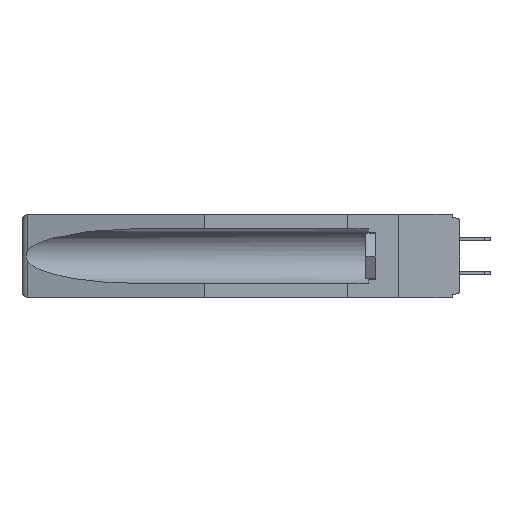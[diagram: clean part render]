
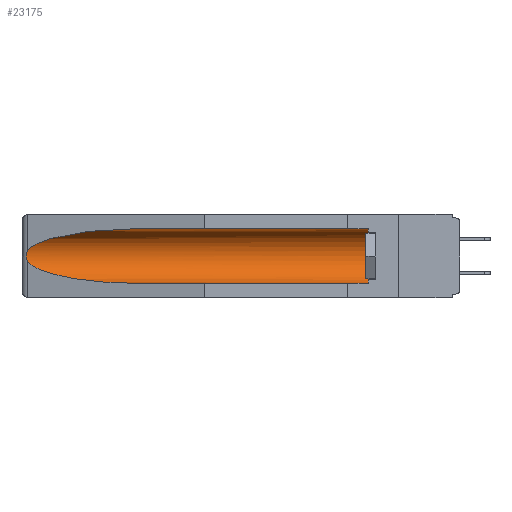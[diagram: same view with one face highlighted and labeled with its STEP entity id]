
A CAD part, left-side view. The second image highlights one B-rep face of the part: STEP entity #23175.
In plain terms, the highlighted cylindrical face has radius 2.857 mm (diameter 5.715 mm), a partial arc.
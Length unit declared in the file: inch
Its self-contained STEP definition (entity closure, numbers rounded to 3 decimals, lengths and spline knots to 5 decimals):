
#35 =( BOUNDED_CURVE ( )  B_SPLINE_CURVE ( 3, ( #17990, #20136, #7535, #20495 ),
 .UNSPECIFIED., .F., .F. ) 
 B_SPLINE_CURVE_WITH_KNOTS ( ( 4, 4 ),
 ( 4.71239, 6.08839 ),
 .UNSPECIFIED. ) 
 CURVE ( )  GEOMETRIC_REPRESENTATION_ITEM ( )  RATIONAL_B_SPLINE_CURVE ( ( 1., 0.848, 0.848, 1. ) ) 
 REPRESENTATION_ITEM ( '' )  );
#2315 = DIRECTION ( 'NONE',  ( 0., 1., 0. ) ) ;
#2699 = CARTESIAN_POINT ( 'NONE',  ( 0.155, -0.30754, -0.1715 ) ) ;
#2771 = ORIENTED_EDGE ( 'NONE', *, *, #7260, .F. ) ;
#3774 = CARTESIAN_POINT ( 'NONE',  ( 0.26654, 1.53092, -0.15636 ) ) ;
#4190 = CARTESIAN_POINT ( 'NONE',  ( 0.26537, 1.52718, -0.14972 ) ) ;
#4200 = CARTESIAN_POINT ( 'NONE',  ( 0.21114, 1.30732, -0.284 ) ) ;
#4686 = ORIENTED_EDGE ( 'NONE', *, *, #25922, .T. ) ;
#4822 = CARTESIAN_POINT ( 'NONE',  ( 0.155, -0.30754, -0.284 ) ) ;
#5340 = EDGE_CURVE ( 'NONE', #10968, #17096, #16891, .T. ) ;
#6312 = LINE ( 'NONE', #21049, #22371 ) ;
#6696 = DIRECTION ( 'NONE',  ( 0., 0., 1. ) ) ;
#7186 = CARTESIAN_POINT ( 'NONE',  ( 0.155, 1.07973, -0.284 ) ) ;
#7260 = EDGE_CURVE ( 'NONE', #10968, #26595, #7734, .T. ) ;
#7535 = CARTESIAN_POINT ( 'NONE',  ( 0.25451, 1.48313, -0.09465 ) ) ;
#7734 = LINE ( 'NONE', #4822, #17746 ) ;
#7871 = CARTESIAN_POINT ( 'NONE',  ( 0.26537, 1.52718, -0.19328 ) ) ;
#7887 = EDGE_CURVE ( 'NONE', #22178, #26595, #15762, .T. ) ;
#8467 = VERTEX_POINT ( 'NONE', #10726 ) ;
#8625 = DIRECTION ( 'NONE',  ( 0., -1., 0. ) ) ;
#9494 = CARTESIAN_POINT ( 'NONE',  ( 0.26597, 1.52961, -0.15275 ) ) ;
#9852 = EDGE_CURVE ( 'NONE', #17096, #8467, #6312, .T. ) ;
#9952 = B_SPLINE_CURVE_WITH_KNOTS ( 'NONE', 3,
 ( #18239, #9494, #3774, #18697, #12110, #27044, #20656, #14518, #16391, #7871 ),
 .UNSPECIFIED., .F., .F.,
 ( 4, 2, 2, 2, 4 ),
 ( 0., 0.00029, 0.00058, 0.00087, 0.00117 ),
 .UNSPECIFIED. ) ;
#10150 = CYLINDRICAL_SURFACE ( 'NONE', #16971, 0.1125 ) ;
#10726 = CARTESIAN_POINT ( 'NONE',  ( 0.155, 1.07973, -0.059 ) ) ;
#10968 = VERTEX_POINT ( 'NONE', #15198 ) ;
#12110 = CARTESIAN_POINT ( 'NONE',  ( 0.2675, 1.53308, -0.16763 ) ) ;
#12717 = AXIS2_PLACEMENT_3D ( 'NONE', #17121, #8625, #19795 ) ;
#14356 = ORIENTED_EDGE ( 'NONE', *, *, #9852, .T. ) ;
#14518 = CARTESIAN_POINT ( 'NONE',  ( 0.26655, 1.53094, -0.18657 ) ) ;
#14848 = CARTESIAN_POINT ( 'NONE',  ( 0.26537, 1.52718, -0.19328 ) ) ;
#15198 = CARTESIAN_POINT ( 'NONE',  ( 0.155, 0.126, -0.284 ) ) ;
#15762 =( BOUNDED_CURVE ( )  B_SPLINE_CURVE ( 3, ( #14848, #16994, #4200, #23515 ),
 .UNSPECIFIED., .F., .F. ) 
 B_SPLINE_CURVE_WITH_KNOTS ( ( 4, 4 ),
 ( 0.1948, 1.5708 ),
 .UNSPECIFIED. ) 
 CURVE ( )  GEOMETRIC_REPRESENTATION_ITEM ( )  RATIONAL_B_SPLINE_CURVE ( ( 1., 0.848, 0.848, 1. ) ) 
 REPRESENTATION_ITEM ( '' )  );
#16153 = FACE_OUTER_BOUND ( 'NONE', #21835, .T. ) ;
#16289 = CARTESIAN_POINT ( 'NONE',  ( 0.26537, 1.52718, -0.19328 ) ) ;
#16391 = CARTESIAN_POINT ( 'NONE',  ( 0.26597, 1.5296, -0.19026 ) ) ;
#16841 = CARTESIAN_POINT ( 'NONE',  ( 0.155, 0.126, -0.059 ) ) ;
#16891 = CIRCLE ( 'NONE', #12717, 0.1125 ) ;
#16971 = AXIS2_PLACEMENT_3D ( 'NONE', #2699, #2315, #6696 ) ;
#16994 = CARTESIAN_POINT ( 'NONE',  ( 0.25451, 1.48313, -0.24835 ) ) ;
#17096 = VERTEX_POINT ( 'NONE', #16841 ) ;
#17121 = CARTESIAN_POINT ( 'NONE',  ( 0.155, 0.126, -0.1715 ) ) ;
#17746 = VECTOR ( 'NONE', #26220, 39.37008 ) ;
#17990 = CARTESIAN_POINT ( 'NONE',  ( 0.155, 1.07973, -0.059 ) ) ;
#18239 = CARTESIAN_POINT ( 'NONE',  ( 0.26537, 1.52718, -0.14972 ) ) ;
#18697 = CARTESIAN_POINT ( 'NONE',  ( 0.2673, 1.5327, -0.16383 ) ) ;
#19138 = EDGE_CURVE ( 'NONE', #25100, #22178, #9952, .T. ) ;
#19795 = DIRECTION ( 'NONE',  ( 0., 0., 1. ) ) ;
#20136 = CARTESIAN_POINT ( 'NONE',  ( 0.21114, 1.30732, -0.059 ) ) ;
#20495 = CARTESIAN_POINT ( 'NONE',  ( 0.26537, 1.52718, -0.14972 ) ) ;
#20656 = CARTESIAN_POINT ( 'NONE',  ( 0.2673, 1.53269, -0.17917 ) ) ;
#21049 = CARTESIAN_POINT ( 'NONE',  ( 0.155, -0.30754, -0.059 ) ) ;
#21835 = EDGE_LOOP ( 'NONE', ( #4686, #23000, #24440, #2771, #21895, #14356 ) ) ;
#21895 = ORIENTED_EDGE ( 'NONE', *, *, #5340, .T. ) ;
#22178 = VERTEX_POINT ( 'NONE', #16289 ) ;
#22371 = VECTOR ( 'NONE', #25481, 39.37008 ) ;
#23000 = ORIENTED_EDGE ( 'NONE', *, *, #19138, .T. ) ;
#23175 = ADVANCED_FACE ( 'NONE', ( #16153 ), #10150, .F. ) ;
#23515 = CARTESIAN_POINT ( 'NONE',  ( 0.155, 1.07973, -0.284 ) ) ;
#24440 = ORIENTED_EDGE ( 'NONE', *, *, #7887, .T. ) ;
#25100 = VERTEX_POINT ( 'NONE', #4190 ) ;
#25481 = DIRECTION ( 'NONE',  ( 0., 1., 0. ) ) ;
#25922 = EDGE_CURVE ( 'NONE', #8467, #25100, #35, .T. ) ;
#26220 = DIRECTION ( 'NONE',  ( 0., 1., 0. ) ) ;
#26595 = VERTEX_POINT ( 'NONE', #7186 ) ;
#27044 = CARTESIAN_POINT ( 'NONE',  ( 0.2675, 1.53308, -0.17534 ) ) ;
